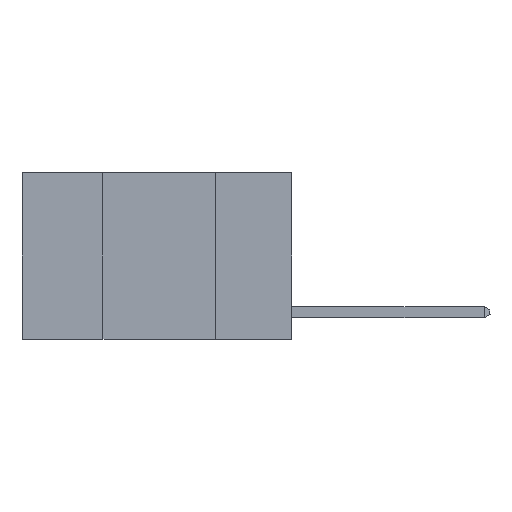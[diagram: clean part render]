
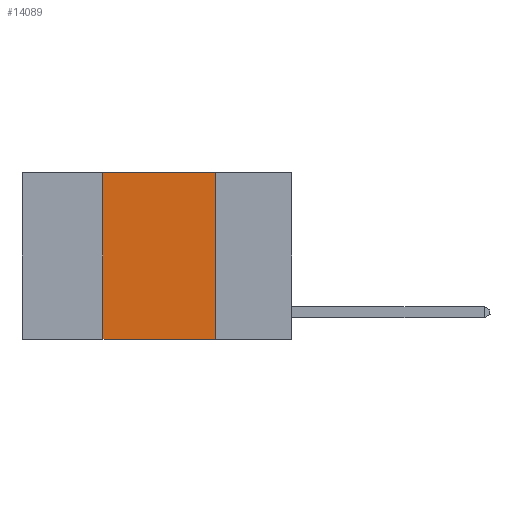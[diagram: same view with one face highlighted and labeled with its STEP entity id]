
A CAD part, left-side view. The second image highlights one B-rep face of the part: STEP entity #14089.
In plain terms, the highlighted planar face has unit normal (-1, 0, 0).
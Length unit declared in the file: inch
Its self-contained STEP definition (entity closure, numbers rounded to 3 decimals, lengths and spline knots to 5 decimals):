
#287 = DIRECTION ( 'NONE',  ( 1., 0., 0. ) ) ;
#892 = CARTESIAN_POINT ( 'NONE',  ( 0., 0.42, 0. ) ) ;
#1368 = VERTEX_POINT ( 'NONE', #21335 ) ;
#1801 = DIRECTION ( 'NONE',  ( 0., -1., 0. ) ) ;
#2354 = ORIENTED_EDGE ( 'NONE', *, *, #5252, .T. ) ;
#4301 = ORIENTED_EDGE ( 'NONE', *, *, #9040, .F. ) ;
#5252 = EDGE_CURVE ( 'NONE', #18948, #17320, #9835, .T. ) ;
#5477 = AXIS2_PLACEMENT_3D ( 'NONE', #18928, #287, #11418 ) ;
#6032 = VERTEX_POINT ( 'NONE', #17438 ) ;
#6794 = ORIENTED_EDGE ( 'NONE', *, *, #8995, .F. ) ;
#6997 = VECTOR ( 'NONE', #23324, 39.37008 ) ;
#8995 = EDGE_CURVE ( 'NONE', #18948, #6032, #19569, .T. ) ;
#9040 = EDGE_CURVE ( 'NONE', #1368, #17320, #10932, .T. ) ;
#9733 = PLANE ( 'NONE',  #5477 ) ;
#9835 = LINE ( 'NONE', #15361, #6997 ) ;
#10462 = DIRECTION ( 'NONE',  ( 0., 0., -1. ) ) ;
#10932 = LINE ( 'NONE', #18452, #13296 ) ;
#11248 = CARTESIAN_POINT ( 'NONE',  ( 0., 0.42, -0.37 ) ) ;
#11418 = DIRECTION ( 'NONE',  ( 0., 0., -1. ) ) ;
#12335 = DIRECTION ( 'NONE',  ( 0., 0., 1. ) ) ;
#12605 = LINE ( 'NONE', #16288, #18628 ) ;
#12889 = VECTOR ( 'NONE', #12335, 39.37008 ) ;
#13296 = VECTOR ( 'NONE', #10462, 39.37008 ) ;
#14089 = ADVANCED_FACE ( 'NONE', ( #21150 ), #9733, .F. ) ;
#15361 = CARTESIAN_POINT ( 'NONE',  ( 0., 0.6, -0.37 ) ) ;
#16288 = CARTESIAN_POINT ( 'NONE',  ( 0., 0.6, 0. ) ) ;
#17320 = VERTEX_POINT ( 'NONE', #22586 ) ;
#17438 = CARTESIAN_POINT ( 'NONE',  ( 0., 0.42, 0. ) ) ;
#18452 = CARTESIAN_POINT ( 'NONE',  ( 0., 0.17, 0. ) ) ;
#18628 = VECTOR ( 'NONE', #1801, 39.37008 ) ;
#18928 = CARTESIAN_POINT ( 'NONE',  ( 0., 0.6, 0. ) ) ;
#18948 = VERTEX_POINT ( 'NONE', #11248 ) ;
#19569 = LINE ( 'NONE', #892, #12889 ) ;
#21150 = FACE_OUTER_BOUND ( 'NONE', #23242, .T. ) ;
#21335 = CARTESIAN_POINT ( 'NONE',  ( 0., 0.17, 0. ) ) ;
#22586 = CARTESIAN_POINT ( 'NONE',  ( 0., 0.17, -0.37 ) ) ;
#22698 = ORIENTED_EDGE ( 'NONE', *, *, #23585, .F. ) ;
#23242 = EDGE_LOOP ( 'NONE', ( #4301, #22698, #6794, #2354 ) ) ;
#23324 = DIRECTION ( 'NONE',  ( 0., -1., 0. ) ) ;
#23585 = EDGE_CURVE ( 'NONE', #6032, #1368, #12605, .T. ) ;
